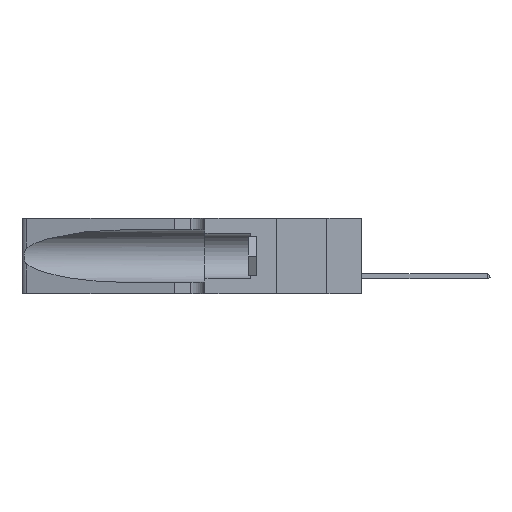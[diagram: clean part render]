
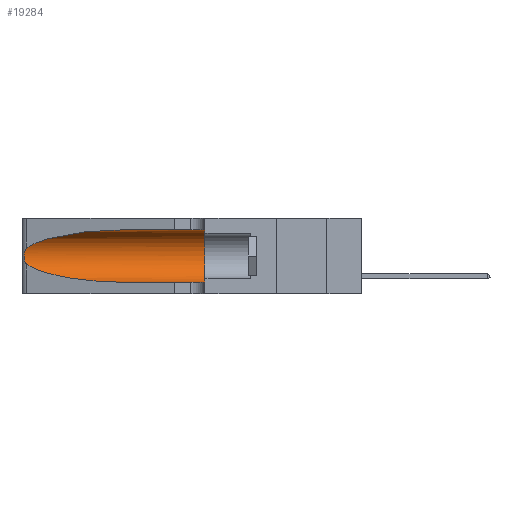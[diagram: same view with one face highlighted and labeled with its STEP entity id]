
A CAD part, left-side view. The second image highlights one B-rep face of the part: STEP entity #19284.
In plain terms, the highlighted cylindrical face has radius 3.308 mm (diameter 6.617 mm), a partial arc.
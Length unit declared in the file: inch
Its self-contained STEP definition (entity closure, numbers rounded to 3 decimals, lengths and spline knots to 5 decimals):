
#170 = CARTESIAN_POINT ( 'NONE',  ( 0.25856, 1.23593, 0.16098 ) ) ;
#286 = DIRECTION ( 'NONE',  ( 0., 0., 1. ) ) ;
#930 = LINE ( 'NONE', #14407, #2162 ) ;
#2001 = LINE ( 'NONE', #16036, #19264 ) ;
#2047 = CARTESIAN_POINT ( 'NONE',  ( 0.25487, 1.22718, 0.22369 ) ) ;
#2162 = VECTOR ( 'NONE', #32602, 39.37008 ) ;
#2558 = CARTESIAN_POINT ( 'NONE',  ( 0.25789, 1.23486, 0.15765 ) ) ;
#4511 = DIRECTION ( 'NONE',  ( 0., 0., -1. ) ) ;
#4573 = FACE_OUTER_BOUND ( 'NONE', #11144, .T. ) ;
#4685 = VERTEX_POINT ( 'NONE', #10944 ) ;
#4722 = DIRECTION ( 'NONE',  ( 0., -1., 0. ) ) ;
#5035 = ORIENTED_EDGE ( 'NONE', *, *, #9061, .F. ) ;
#5582 = B_SPLINE_CURVE_WITH_KNOTS ( 'NONE', 3,
 ( #25340, #30179, #30290, #23260, #17986, #10440, #33267, #15413, #7855, #170, #2558, #25747, #31008, #30809 ),
 .UNSPECIFIED., .F., .F.,
 ( 4, 2, 2, 2, 2, 2, 4 ),
 ( 0., 0.00027, 0.00053, 0.00107, 0.0016, 0.00187, 0.00214 ),
 .UNSPECIFIED. ) ;
#5951 = AXIS2_PLACEMENT_3D ( 'NONE', #31595, #33054, #286 ) ;
#6717 = EDGE_CURVE ( 'NONE', #16552, #12133, #31884, .T. ) ;
#7855 = CARTESIAN_POINT ( 'NONE',  ( 0.26017, 1.23833, 0.17102 ) ) ;
#9061 = EDGE_CURVE ( 'NONE', #17853, #16552, #930, .T. ) ;
#9215 = ORIENTED_EDGE ( 'NONE', *, *, #15231, .T. ) ;
#10284 = ORIENTED_EDGE ( 'NONE', *, *, #28437, .T. ) ;
#10440 = CARTESIAN_POINT ( 'NONE',  ( 0.26018, 1.23835, 0.19895 ) ) ;
#10944 = CARTESIAN_POINT ( 'NONE',  ( 0.1305, 0.72297, 0.05475 ) ) ;
#11018 = CARTESIAN_POINT ( 'NONE',  ( 0.18966, 0.96281, 0.05475 ) ) ;
#11033 = CARTESIAN_POINT ( 'NONE',  ( 0.1305, 0.35, 0.31525 ) ) ;
#11144 = EDGE_LOOP ( 'NONE', ( #14329, #10284, #9215, #23901, #13992, #5035 ) ) ;
#11621 =( BOUNDED_CURVE ( )  B_SPLINE_CURVE ( 3, ( #15978, #31059, #20921, #28829 ),
 .UNSPECIFIED., .F., .F. ) 
 B_SPLINE_CURVE_WITH_KNOTS ( ( 4, 4 ),
 ( 1.5708, 2.84003 ),
 .UNSPECIFIED. ) 
 CURVE ( )  GEOMETRIC_REPRESENTATION_ITEM ( )  RATIONAL_B_SPLINE_CURVE ( ( 1., 0.87, 0.87, 1. ) ) 
 REPRESENTATION_ITEM ( '' )  );
#11838 = CARTESIAN_POINT ( 'NONE',  ( 0.1305, 1.61858, 0.185 ) ) ;
#12133 = VERTEX_POINT ( 'NONE', #23940 ) ;
#12724 =( BOUNDED_CURVE ( )  B_SPLINE_CURVE ( 3, ( #32558, #14690, #11018, #25282 ),
 .UNSPECIFIED., .F., .F. ) 
 B_SPLINE_CURVE_WITH_KNOTS ( ( 4, 4 ),
 ( 3.44316, 4.71239 ),
 .UNSPECIFIED. ) 
 CURVE ( )  GEOMETRIC_REPRESENTATION_ITEM ( )  RATIONAL_B_SPLINE_CURVE ( ( 1., 0.87, 0.87, 1. ) ) 
 REPRESENTATION_ITEM ( '' )  );
#13229 = VERTEX_POINT ( 'NONE', #2047 ) ;
#13992 = ORIENTED_EDGE ( 'NONE', *, *, #6717, .F. ) ;
#14329 = ORIENTED_EDGE ( 'NONE', *, *, #23229, .T. ) ;
#14407 = CARTESIAN_POINT ( 'NONE',  ( 0.1305, 1.61858, 0.31525 ) ) ;
#14690 = CARTESIAN_POINT ( 'NONE',  ( 0.2373, 1.15595, 0.08982 ) ) ;
#15231 = EDGE_CURVE ( 'NONE', #19206, #4685, #12724, .T. ) ;
#15413 = CARTESIAN_POINT ( 'NONE',  ( 0.26075, 1.23896, 0.178 ) ) ;
#15978 = CARTESIAN_POINT ( 'NONE',  ( 0.1305, 0.72297, 0.31525 ) ) ;
#16036 = CARTESIAN_POINT ( 'NONE',  ( 0.1305, 1.61858, 0.05475 ) ) ;
#16552 = VERTEX_POINT ( 'NONE', #11033 ) ;
#17853 = VERTEX_POINT ( 'NONE', #27995 ) ;
#17986 = CARTESIAN_POINT ( 'NONE',  ( 0.25854, 1.2359, 0.20912 ) ) ;
#19206 = VERTEX_POINT ( 'NONE', #31478 ) ;
#19264 = VECTOR ( 'NONE', #21865, 39.37008 ) ;
#19284 = ADVANCED_FACE ( 'NONE', ( #4573 ), #25121, .F. ) ;
#20921 = CARTESIAN_POINT ( 'NONE',  ( 0.2373, 1.15595, 0.28018 ) ) ;
#21865 = DIRECTION ( 'NONE',  ( 0., -1., 0. ) ) ;
#23229 = EDGE_CURVE ( 'NONE', #17853, #13229, #11621, .T. ) ;
#23260 = CARTESIAN_POINT ( 'NONE',  ( 0.25787, 1.23484, 0.2124 ) ) ;
#23901 = ORIENTED_EDGE ( 'NONE', *, *, #28665, .T. ) ;
#23940 = CARTESIAN_POINT ( 'NONE',  ( 0.1305, 0.35, 0.05475 ) ) ;
#25121 = CYLINDRICAL_SURFACE ( 'NONE', #25492, 0.13025 ) ;
#25282 = CARTESIAN_POINT ( 'NONE',  ( 0.1305, 0.72297, 0.05475 ) ) ;
#25340 = CARTESIAN_POINT ( 'NONE',  ( 0.25487, 1.22718, 0.22369 ) ) ;
#25492 = AXIS2_PLACEMENT_3D ( 'NONE', #11838, #4722, #4511 ) ;
#25747 = CARTESIAN_POINT ( 'NONE',  ( 0.25639, 1.23186, 0.15144 ) ) ;
#27995 = CARTESIAN_POINT ( 'NONE',  ( 0.1305, 0.72297, 0.31525 ) ) ;
#28437 = EDGE_CURVE ( 'NONE', #13229, #19206, #5582, .T. ) ;
#28665 = EDGE_CURVE ( 'NONE', #4685, #12133, #2001, .T. ) ;
#28829 = CARTESIAN_POINT ( 'NONE',  ( 0.25487, 1.22718, 0.22369 ) ) ;
#30179 = CARTESIAN_POINT ( 'NONE',  ( 0.25555, 1.22994, 0.2215 ) ) ;
#30290 = CARTESIAN_POINT ( 'NONE',  ( 0.25639, 1.23184, 0.21858 ) ) ;
#30809 = CARTESIAN_POINT ( 'NONE',  ( 0.25487, 1.22718, 0.14631 ) ) ;
#31008 = CARTESIAN_POINT ( 'NONE',  ( 0.25555, 1.22993, 0.14849 ) ) ;
#31059 = CARTESIAN_POINT ( 'NONE',  ( 0.18966, 0.96281, 0.31525 ) ) ;
#31478 = CARTESIAN_POINT ( 'NONE',  ( 0.25487, 1.22718, 0.14631 ) ) ;
#31595 = CARTESIAN_POINT ( 'NONE',  ( 0.1305, 0.35, 0.185 ) ) ;
#31884 = CIRCLE ( 'NONE', #5951, 0.13025 ) ;
#32558 = CARTESIAN_POINT ( 'NONE',  ( 0.25487, 1.22718, 0.14631 ) ) ;
#32602 = DIRECTION ( 'NONE',  ( 0., -1., 0. ) ) ;
#33054 = DIRECTION ( 'NONE',  ( 0., 1., 0. ) ) ;
#33267 = CARTESIAN_POINT ( 'NONE',  ( 0.26075, 1.23896, 0.19203 ) ) ;
